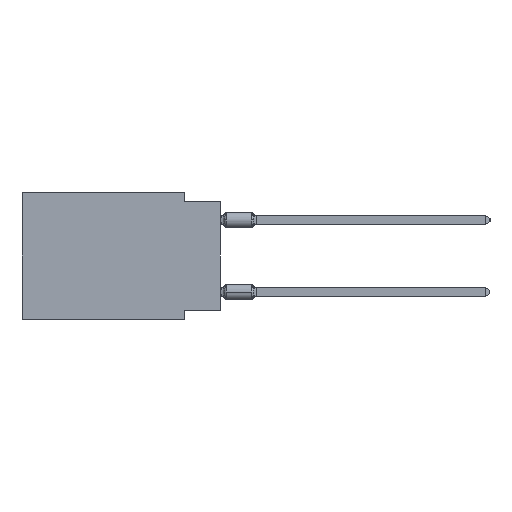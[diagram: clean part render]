
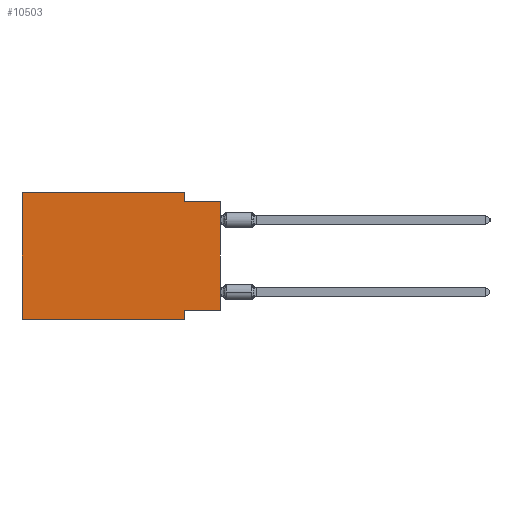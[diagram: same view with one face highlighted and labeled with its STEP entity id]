
A CAD part, left-side view. The second image highlights one B-rep face of the part: STEP entity #10503.
In plain terms, the highlighted planar face has unit normal (-1, 0, 0).
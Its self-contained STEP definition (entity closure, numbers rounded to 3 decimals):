
#1162 = FACE_OUTER_BOUND ( 'NONE', #23713, .T. ) ;
#1908 = DIRECTION ( 'NONE',  ( 1., 0., 0. ) ) ;
#2189 = CARTESIAN_POINT ( 'NONE',  ( 0., 2.54, 0. ) ) ;
#2381 = VERTEX_POINT ( 'NONE', #49431 ) ;
#3613 = CARTESIAN_POINT ( 'NONE',  ( 0., 13.97, 0. ) ) ;
#5903 = VERTEX_POINT ( 'NONE', #2189 ) ;
#6635 = CARTESIAN_POINT ( 'NONE',  ( 0., 13.97, 0. ) ) ;
#7692 = EDGE_CURVE ( 'NONE', #55738, #14185, #51405, .T. ) ;
#9315 = VECTOR ( 'NONE', #62673, 1000. ) ;
#10130 = VECTOR ( 'NONE', #40879, 1000. ) ;
#10285 = CARTESIAN_POINT ( 'NONE',  ( 0., 2.54, -8.89 ) ) ;
#10503 = ADVANCED_FACE ( 'NONE', ( #1162 ), #29817, .F. ) ;
#10533 = ORIENTED_EDGE ( 'NONE', *, *, #58689, .F. ) ;
#10596 = CARTESIAN_POINT ( 'NONE',  ( 0., 2.54, -8.255 ) ) ;
#10661 = LINE ( 'NONE', #50876, #19578 ) ;
#14101 = EDGE_CURVE ( 'NONE', #31136, #2381, #10661, .T. ) ;
#14185 = VERTEX_POINT ( 'NONE', #10285 ) ;
#15057 = VECTOR ( 'NONE', #21387, 1000. ) ;
#16624 = DIRECTION ( 'NONE',  ( 0., -1., 0. ) ) ;
#18160 = LINE ( 'NONE', #6635, #10130 ) ;
#19155 = DIRECTION ( 'NONE',  ( 0., 0., 1. ) ) ;
#19578 = VECTOR ( 'NONE', #16624, 1000. ) ;
#19821 = VERTEX_POINT ( 'NONE', #3613 ) ;
#19832 = EDGE_CURVE ( 'NONE', #52839, #55738, #32283, .T. ) ;
#21084 = CARTESIAN_POINT ( 'NONE',  ( 0., 2.54, 0. ) ) ;
#21387 = DIRECTION ( 'NONE',  ( 0., -1., 0. ) ) ;
#22012 = AXIS2_PLACEMENT_3D ( 'NONE', #34673, #1908, #30555 ) ;
#23482 = ORIENTED_EDGE ( 'NONE', *, *, #19832, .F. ) ;
#23657 = EDGE_CURVE ( 'NONE', #58778, #14185, #65699, .T. ) ;
#23713 = EDGE_LOOP ( 'NONE', ( #34508, #53770, #54568, #10533, #24538, #25237, #36541, #23482 ) ) ;
#23838 = CARTESIAN_POINT ( 'NONE',  ( 0., 2.54, -8.89 ) ) ;
#24538 = ORIENTED_EDGE ( 'NONE', *, *, #27102, .F. ) ;
#25237 = ORIENTED_EDGE ( 'NONE', *, *, #23657, .T. ) ;
#27102 = EDGE_CURVE ( 'NONE', #58778, #19821, #18160, .T. ) ;
#29817 = PLANE ( 'NONE',  #22012 ) ;
#30555 = DIRECTION ( 'NONE',  ( 0., 0., -1. ) ) ;
#31136 = VERTEX_POINT ( 'NONE', #69777 ) ;
#32283 = LINE ( 'NONE', #51500, #9315 ) ;
#33195 = CARTESIAN_POINT ( 'NONE',  ( 0., 13.97, 0. ) ) ;
#34508 = ORIENTED_EDGE ( 'NONE', *, *, #50974, .T. ) ;
#34673 = CARTESIAN_POINT ( 'NONE',  ( 0., 13.97, 0. ) ) ;
#34812 = CARTESIAN_POINT ( 'NONE',  ( 0., 0., 0. ) ) ;
#35763 = CARTESIAN_POINT ( 'NONE',  ( 0., 13.97, -8.89 ) ) ;
#36541 = ORIENTED_EDGE ( 'NONE', *, *, #7692, .F. ) ;
#38028 = CARTESIAN_POINT ( 'NONE',  ( 0., 0., -8.255 ) ) ;
#38358 = VECTOR ( 'NONE', #44737, 1000. ) ;
#38472 = VECTOR ( 'NONE', #46548, 1000. ) ;
#40879 = DIRECTION ( 'NONE',  ( 0., 0., 1. ) ) ;
#41084 = EDGE_CURVE ( 'NONE', #5903, #31136, #59807, .T. ) ;
#44737 = DIRECTION ( 'NONE',  ( 0., -1., 0. ) ) ;
#46548 = DIRECTION ( 'NONE',  ( 0., 0., -1. ) ) ;
#48144 = VECTOR ( 'NONE', #19155, 1000. ) ;
#49431 = CARTESIAN_POINT ( 'NONE',  ( 0., 0., -0.635 ) ) ;
#50876 = CARTESIAN_POINT ( 'NONE',  ( 0., 0., -0.635 ) ) ;
#50974 = EDGE_CURVE ( 'NONE', #52839, #2381, #69046, .T. ) ;
#51405 = LINE ( 'NONE', #23838, #38472 ) ;
#51500 = CARTESIAN_POINT ( 'NONE',  ( 0., 0., -8.255 ) ) ;
#52839 = VERTEX_POINT ( 'NONE', #38028 ) ;
#53770 = ORIENTED_EDGE ( 'NONE', *, *, #14101, .F. ) ;
#54568 = ORIENTED_EDGE ( 'NONE', *, *, #41084, .F. ) ;
#55738 = VERTEX_POINT ( 'NONE', #10596 ) ;
#58689 = EDGE_CURVE ( 'NONE', #19821, #5903, #66332, .T. ) ;
#58778 = VERTEX_POINT ( 'NONE', #35763 ) ;
#59221 = VECTOR ( 'NONE', #60904, 1000. ) ;
#59807 = LINE ( 'NONE', #21084, #59221 ) ;
#60904 = DIRECTION ( 'NONE',  ( 0., 0., -1. ) ) ;
#62673 = DIRECTION ( 'NONE',  ( 0., 1., 0. ) ) ;
#65699 = LINE ( 'NONE', #70909, #15057 ) ;
#66332 = LINE ( 'NONE', #33195, #38358 ) ;
#69046 = LINE ( 'NONE', #34812, #48144 ) ;
#69777 = CARTESIAN_POINT ( 'NONE',  ( 0., 2.54, -0.635 ) ) ;
#70909 = CARTESIAN_POINT ( 'NONE',  ( 0., 13.97, -8.89 ) ) ;
